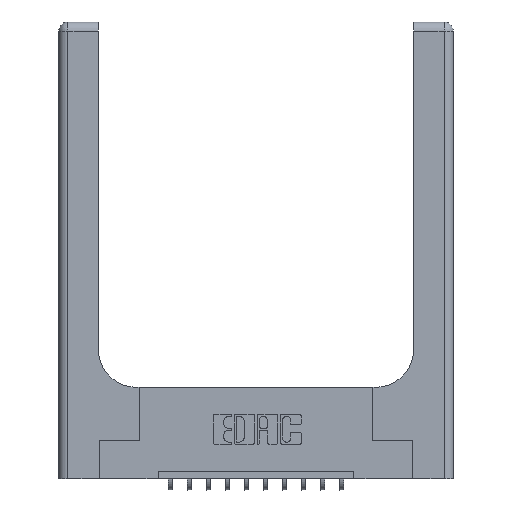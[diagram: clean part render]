
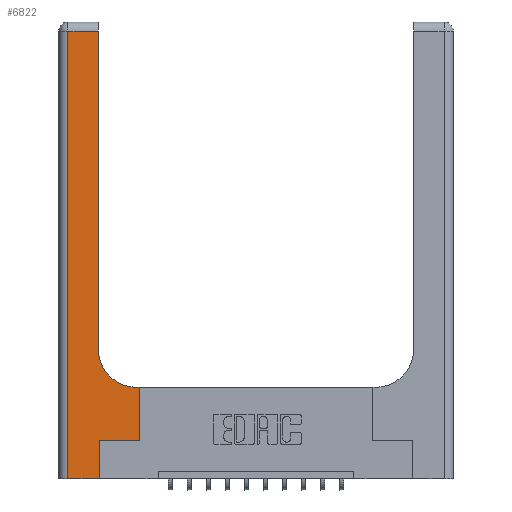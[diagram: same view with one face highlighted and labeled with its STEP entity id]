
A CAD part, top view. The second image highlights one B-rep face of the part: STEP entity #6822.
In plain terms, the highlighted planar face has unit normal (0, 0, 1).
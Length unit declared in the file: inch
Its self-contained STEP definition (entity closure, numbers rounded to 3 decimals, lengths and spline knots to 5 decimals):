
#322 = CARTESIAN_POINT ( 'NONE',  ( 0.528, 0.25, 0.37 ) ) ;
#447 = ORIENTED_EDGE ( 'NONE', *, *, #5091, .T. ) ;
#773 = VERTEX_POINT ( 'NONE', #322 ) ;
#1057 = VERTEX_POINT ( 'NONE', #7762 ) ;
#1369 = LINE ( 'NONE', #7659, #4216 ) ;
#2076 = EDGE_CURVE ( 'NONE', #1057, #12098, #2887, .T. ) ;
#2157 = FACE_OUTER_BOUND ( 'NONE', #3840, .T. ) ;
#2377 = VERTEX_POINT ( 'NONE', #16047 ) ;
#2408 = LINE ( 'NONE', #11199, #6171 ) ;
#2501 = CARTESIAN_POINT ( 'NONE',  ( 0.528, 0.25, 0.37 ) ) ;
#2691 = EDGE_CURVE ( 'NONE', #9966, #773, #2408, .T. ) ;
#2887 = CIRCLE ( 'NONE', #11536, 0.25 ) ;
#2947 = EDGE_CURVE ( 'NONE', #12953, #9133, #8209, .T. ) ;
#3026 = DIRECTION ( 'NONE',  ( 1., 0., 0. ) ) ;
#3359 = CARTESIAN_POINT ( 'NONE',  ( 0.265, 0., 0.37 ) ) ;
#3521 = DIRECTION ( 'NONE',  ( 0., -1., 0. ) ) ;
#3792 = ORIENTED_EDGE ( 'NONE', *, *, #14281, .T. ) ;
#3840 = EDGE_LOOP ( 'NONE', ( #447, #15094, #15565, #3792, #9221, #11439, #4059, #15952, #10616 ) ) ;
#4014 = CARTESIAN_POINT ( 'NONE',  ( 0.06, 2.94, 0.37 ) ) ;
#4059 = ORIENTED_EDGE ( 'NONE', *, *, #9319, .T. ) ;
#4216 = VECTOR ( 'NONE', #7502, 39.37008 ) ;
#4485 = CARTESIAN_POINT ( 'NONE',  ( 0.26, 0.85, 0.37 ) ) ;
#5091 = EDGE_CURVE ( 'NONE', #12098, #2377, #10724, .T. ) ;
#5177 = DIRECTION ( 'NONE',  ( 1., 0., 0. ) ) ;
#5688 = VECTOR ( 'NONE', #15983, 39.37008 ) ;
#6171 = VECTOR ( 'NONE', #5177, 39.37008 ) ;
#6478 = CARTESIAN_POINT ( 'NONE',  ( 0.265, 0., 0.37 ) ) ;
#6822 = ADVANCED_FACE ( 'NONE', ( #2157 ), #12168, .F. ) ;
#7502 = DIRECTION ( 'NONE',  ( -1., 0., 0. ) ) ;
#7659 = CARTESIAN_POINT ( 'NONE',  ( 0., 2.94, 0.37 ) ) ;
#7710 = EDGE_CURVE ( 'NONE', #2377, #12953, #1369, .T. ) ;
#7762 = CARTESIAN_POINT ( 'NONE',  ( 0.51, 0.6, 0.37 ) ) ;
#8099 = DIRECTION ( 'NONE',  ( 0., 0., -1. ) ) ;
#8177 = CARTESIAN_POINT ( 'NONE',  ( 0.51, 0.85, 0.37 ) ) ;
#8209 = LINE ( 'NONE', #14611, #8447 ) ;
#8447 = VECTOR ( 'NONE', #3521, 39.37008 ) ;
#8722 = DIRECTION ( 'NONE',  ( 1., 0., 0. ) ) ;
#9133 = VERTEX_POINT ( 'NONE', #15789 ) ;
#9221 = ORIENTED_EDGE ( 'NONE', *, *, #16210, .T. ) ;
#9307 = DIRECTION ( 'NONE',  ( -1., 0., 0. ) ) ;
#9319 = EDGE_CURVE ( 'NONE', #773, #9343, #11375, .T. ) ;
#9343 = VERTEX_POINT ( 'NONE', #11047 ) ;
#9628 = CARTESIAN_POINT ( 'NONE',  ( 0.26, 0.6, 0.37 ) ) ;
#9966 = VERTEX_POINT ( 'NONE', #14577 ) ;
#10058 = CARTESIAN_POINT ( 'NONE',  ( 0., 0., 0.37 ) ) ;
#10616 = ORIENTED_EDGE ( 'NONE', *, *, #2076, .T. ) ;
#10646 = VECTOR ( 'NONE', #8722, 39.37008 ) ;
#10724 = LINE ( 'NONE', #14328, #10939 ) ;
#10939 = VECTOR ( 'NONE', #14398, 39.37008 ) ;
#11047 = CARTESIAN_POINT ( 'NONE',  ( 0.528, 0.6, 0.37 ) ) ;
#11118 = EDGE_CURVE ( 'NONE', #9343, #1057, #12086, .T. ) ;
#11199 = CARTESIAN_POINT ( 'NONE',  ( 0.265, 0.25, 0.37 ) ) ;
#11375 = LINE ( 'NONE', #2501, #12662 ) ;
#11439 = ORIENTED_EDGE ( 'NONE', *, *, #2691, .T. ) ;
#11478 = VERTEX_POINT ( 'NONE', #6478 ) ;
#11536 = AXIS2_PLACEMENT_3D ( 'NONE', #8177, #8099, #3026 ) ;
#11861 = AXIS2_PLACEMENT_3D ( 'NONE', #12011, #15923, #13248 ) ;
#12011 = CARTESIAN_POINT ( 'NONE',  ( 0., 3., 0.37 ) ) ;
#12086 = LINE ( 'NONE', #9628, #14529 ) ;
#12098 = VERTEX_POINT ( 'NONE', #4485 ) ;
#12168 = PLANE ( 'NONE',  #11861 ) ;
#12237 = LINE ( 'NONE', #3359, #5688 ) ;
#12662 = VECTOR ( 'NONE', #14880, 39.37008 ) ;
#12953 = VERTEX_POINT ( 'NONE', #4014 ) ;
#13248 = DIRECTION ( 'NONE',  ( -1., 0., 0. ) ) ;
#14281 = EDGE_CURVE ( 'NONE', #9133, #11478, #14878, .T. ) ;
#14328 = CARTESIAN_POINT ( 'NONE',  ( 0.26, 3., 0.37 ) ) ;
#14398 = DIRECTION ( 'NONE',  ( 0., 1., 0. ) ) ;
#14529 = VECTOR ( 'NONE', #9307, 39.37008 ) ;
#14577 = CARTESIAN_POINT ( 'NONE',  ( 0.265, 0.25, 0.37 ) ) ;
#14611 = CARTESIAN_POINT ( 'NONE',  ( 0.06, 3., 0.37 ) ) ;
#14878 = LINE ( 'NONE', #10058, #10646 ) ;
#14880 = DIRECTION ( 'NONE',  ( 0., 1., 0. ) ) ;
#15094 = ORIENTED_EDGE ( 'NONE', *, *, #7710, .T. ) ;
#15565 = ORIENTED_EDGE ( 'NONE', *, *, #2947, .T. ) ;
#15789 = CARTESIAN_POINT ( 'NONE',  ( 0.06, 0., 0.37 ) ) ;
#15923 = DIRECTION ( 'NONE',  ( 0., 0., -1. ) ) ;
#15952 = ORIENTED_EDGE ( 'NONE', *, *, #11118, .T. ) ;
#15983 = DIRECTION ( 'NONE',  ( 0., 1., 0. ) ) ;
#16047 = CARTESIAN_POINT ( 'NONE',  ( 0.26, 2.94, 0.37 ) ) ;
#16210 = EDGE_CURVE ( 'NONE', #11478, #9966, #12237, .T. ) ;
